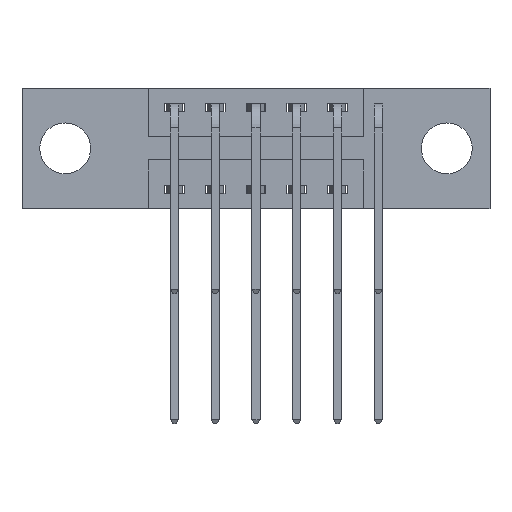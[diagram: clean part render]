
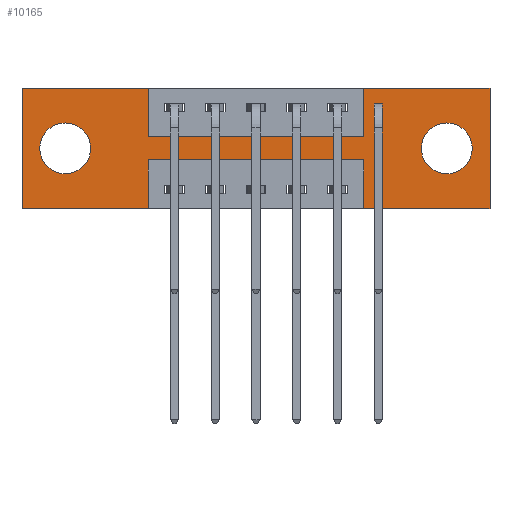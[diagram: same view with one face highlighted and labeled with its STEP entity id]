
A CAD part, front view. The second image highlights one B-rep face of the part: STEP entity #10165.
In plain terms, the highlighted planar face has unit normal (0, -1, 0).
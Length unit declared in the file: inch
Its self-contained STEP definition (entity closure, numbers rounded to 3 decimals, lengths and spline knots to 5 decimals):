
#234 = CARTESIAN_POINT ( 'NONE',  ( 0., 0., 0. ) ) ;
#360 = ORIENTED_EDGE ( 'NONE', *, *, #2505, .F. ) ;
#414 = DIRECTION ( 'NONE',  ( 0., 1., 0. ) ) ;
#424 = VECTOR ( 'NONE', #8199, 39.37008 ) ;
#481 = AXIS2_PLACEMENT_3D ( 'NONE', #708, #5631, #4730 ) ;
#499 = CIRCLE ( 'NONE', #2351, 0.078 ) ;
#577 = ORIENTED_EDGE ( 'NONE', *, *, #3240, .F. ) ;
#701 = ORIENTED_EDGE ( 'NONE', *, *, #3460, .T. ) ;
#708 = CARTESIAN_POINT ( 'NONE',  ( 0.1325, 0., -0.185 ) ) ;
#814 = EDGE_CURVE ( 'NONE', #5803, #1529, #7982, .T. ) ;
#855 = CARTESIAN_POINT ( 'NONE',  ( 0.3875, 0., 0. ) ) ;
#901 = ORIENTED_EDGE ( 'NONE', *, *, #8834, .F. ) ;
#1125 = EDGE_CURVE ( 'NONE', #2244, #5803, #10156, .T. ) ;
#1175 = DIRECTION ( 'NONE',  ( 0., 0., 1. ) ) ;
#1184 = DIRECTION ( 'NONE',  ( 1., 0., 0. ) ) ;
#1345 = DIRECTION ( 'NONE',  ( 0., 0., -1. ) ) ;
#1442 = CARTESIAN_POINT ( 'NONE',  ( 0.3875, 0., -0.37 ) ) ;
#1457 = CARTESIAN_POINT ( 'NONE',  ( 0.3875, 0., -0.15 ) ) ;
#1469 = CARTESIAN_POINT ( 'NONE',  ( 0., 0., 0. ) ) ;
#1529 = VERTEX_POINT ( 'NONE', #6823 ) ;
#1663 = CARTESIAN_POINT ( 'NONE',  ( 0., 0., -0.37 ) ) ;
#1689 = EDGE_LOOP ( 'NONE', ( #5128, #8986, #4815, #3028, #5295, #10006, #360, #7172, #8598, #577, #7775, #901 ) ) ;
#1960 = DIRECTION ( 'NONE',  ( 0., 1., 0. ) ) ;
#1968 = EDGE_CURVE ( 'NONE', #5763, #8391, #9096, .T. ) ;
#2097 = EDGE_CURVE ( 'NONE', #4335, #2244, #2822, .T. ) ;
#2244 = VERTEX_POINT ( 'NONE', #7338 ) ;
#2286 = EDGE_CURVE ( 'NONE', #3604, #5763, #9835, .T. ) ;
#2351 = AXIS2_PLACEMENT_3D ( 'NONE', #7688, #414, #3644 ) ;
#2410 = EDGE_LOOP ( 'NONE', ( #7696, #3784 ) ) ;
#2499 = VECTOR ( 'NONE', #6369, 39.37008 ) ;
#2505 = EDGE_CURVE ( 'NONE', #8391, #4384, #7104, .T. ) ;
#2518 = VECTOR ( 'NONE', #7050, 39.37008 ) ;
#2637 = VERTEX_POINT ( 'NONE', #1663 ) ;
#2639 = CARTESIAN_POINT ( 'NONE',  ( 0., 0., -0.37 ) ) ;
#2676 = VECTOR ( 'NONE', #4976, 39.37008 ) ;
#2822 = LINE ( 'NONE', #3824, #2499 ) ;
#2904 = VECTOR ( 'NONE', #5987, 39.37008 ) ;
#2987 = LINE ( 'NONE', #1442, #7530 ) ;
#3028 = ORIENTED_EDGE ( 'NONE', *, *, #1125, .F. ) ;
#3036 = CARTESIAN_POINT ( 'NONE',  ( 0.3875, 0., -0.22 ) ) ;
#3152 = CARTESIAN_POINT ( 'NONE',  ( 0., 0., -0.37 ) ) ;
#3240 = EDGE_CURVE ( 'NONE', #6927, #3604, #7519, .T. ) ;
#3460 = EDGE_CURVE ( 'NONE', #4185, #4206, #8150, .T. ) ;
#3530 = CARTESIAN_POINT ( 'NONE',  ( 1.3025, 0., -0.263 ) ) ;
#3537 = DIRECTION ( 'NONE',  ( -1., 0., 0. ) ) ;
#3566 = VECTOR ( 'NONE', #1184, 39.37008 ) ;
#3604 = VERTEX_POINT ( 'NONE', #5953 ) ;
#3644 = DIRECTION ( 'NONE',  ( 0., 0., -1. ) ) ;
#3784 = ORIENTED_EDGE ( 'NONE', *, *, #6646, .T. ) ;
#3816 = LINE ( 'NONE', #1469, #2518 ) ;
#3823 = CARTESIAN_POINT ( 'NONE',  ( 1.0475, 0., -0.37 ) ) ;
#3824 = CARTESIAN_POINT ( 'NONE',  ( 1.435, 0., 0. ) ) ;
#3940 = EDGE_LOOP ( 'NONE', ( #8589, #701 ) ) ;
#3952 = LINE ( 'NONE', #3152, #424 ) ;
#4122 = CARTESIAN_POINT ( 'NONE',  ( 0., 0., 0. ) ) ;
#4185 = VERTEX_POINT ( 'NONE', #3530 ) ;
#4206 = VERTEX_POINT ( 'NONE', #6722 ) ;
#4335 = VERTEX_POINT ( 'NONE', #9390 ) ;
#4384 = VERTEX_POINT ( 'NONE', #6299 ) ;
#4392 = LINE ( 'NONE', #10049, #2904 ) ;
#4565 = VECTOR ( 'NONE', #9618, 39.37008 ) ;
#4673 = AXIS2_PLACEMENT_3D ( 'NONE', #9257, #1960, #1175 ) ;
#4730 = DIRECTION ( 'NONE',  ( 0., 0., 1. ) ) ;
#4815 = ORIENTED_EDGE ( 'NONE', *, *, #814, .F. ) ;
#4856 = VECTOR ( 'NONE', #10333, 39.37008 ) ;
#4886 = DIRECTION ( 'NONE',  ( 0., 0., -1. ) ) ;
#4976 = DIRECTION ( 'NONE',  ( 0., 0., -1. ) ) ;
#5051 = CIRCLE ( 'NONE', #481, 0.078 ) ;
#5128 = ORIENTED_EDGE ( 'NONE', *, *, #7564, .F. ) ;
#5209 = VECTOR ( 'NONE', #3537, 39.37008 ) ;
#5295 = ORIENTED_EDGE ( 'NONE', *, *, #2097, .F. ) ;
#5406 = FACE_OUTER_BOUND ( 'NONE', #1689, .T. ) ;
#5475 = AXIS2_PLACEMENT_3D ( 'NONE', #7860, #8645, #10265 ) ;
#5510 = FACE_BOUND ( 'NONE', #2410, .T. ) ;
#5631 = DIRECTION ( 'NONE',  ( 0., 1., 0. ) ) ;
#5763 = VERTEX_POINT ( 'NONE', #1457 ) ;
#5803 = VERTEX_POINT ( 'NONE', #8009 ) ;
#5953 = CARTESIAN_POINT ( 'NONE',  ( 0.3875, 0., 0. ) ) ;
#5987 = DIRECTION ( 'NONE',  ( -1., 0., 0. ) ) ;
#6076 = EDGE_CURVE ( 'NONE', #2637, #6927, #9760, .T. ) ;
#6196 = CIRCLE ( 'NONE', #4673, 0.078 ) ;
#6202 = VECTOR ( 'NONE', #9002, 39.37008 ) ;
#6299 = CARTESIAN_POINT ( 'NONE',  ( 1.0475, 0., 0. ) ) ;
#6369 = DIRECTION ( 'NONE',  ( 0., 0., -1. ) ) ;
#6541 = DIRECTION ( 'NONE',  ( 0., 1., 0. ) ) ;
#6641 = VERTEX_POINT ( 'NONE', #7672 ) ;
#6646 = EDGE_CURVE ( 'NONE', #6641, #9813, #6196, .T. ) ;
#6722 = CARTESIAN_POINT ( 'NONE',  ( 1.3025, 0., -0.107 ) ) ;
#6823 = CARTESIAN_POINT ( 'NONE',  ( 1.0475, 0., -0.22 ) ) ;
#6927 = VERTEX_POINT ( 'NONE', #7342 ) ;
#6934 = CARTESIAN_POINT ( 'NONE',  ( 0.1325, 0., -0.107 ) ) ;
#6960 = AXIS2_PLACEMENT_3D ( 'NONE', #7240, #6541, #4886 ) ;
#7050 = DIRECTION ( 'NONE',  ( 1., 0., 0. ) ) ;
#7104 = LINE ( 'NONE', #7212, #4565 ) ;
#7172 = ORIENTED_EDGE ( 'NONE', *, *, #1968, .F. ) ;
#7212 = CARTESIAN_POINT ( 'NONE',  ( 1.0475, 0., 0. ) ) ;
#7240 = CARTESIAN_POINT ( 'NONE',  ( 1.3025, 0., -0.185 ) ) ;
#7338 = CARTESIAN_POINT ( 'NONE',  ( 1.435, 0., -0.37 ) ) ;
#7342 = CARTESIAN_POINT ( 'NONE',  ( 0., 0., 0. ) ) ;
#7375 = CARTESIAN_POINT ( 'NONE',  ( 1.0475, 0., -0.15 ) ) ;
#7418 = CARTESIAN_POINT ( 'NONE',  ( 0.3875, 0., -0.15 ) ) ;
#7519 = LINE ( 'NONE', #234, #3566 ) ;
#7530 = VECTOR ( 'NONE', #1345, 39.37008 ) ;
#7564 = EDGE_CURVE ( 'NONE', #9030, #8965, #2987, .T. ) ;
#7672 = CARTESIAN_POINT ( 'NONE',  ( 0.1325, 0., -0.263 ) ) ;
#7688 = CARTESIAN_POINT ( 'NONE',  ( 1.3025, 0., -0.185 ) ) ;
#7696 = ORIENTED_EDGE ( 'NONE', *, *, #9245, .T. ) ;
#7775 = ORIENTED_EDGE ( 'NONE', *, *, #6076, .F. ) ;
#7860 = CARTESIAN_POINT ( 'NONE',  ( 0., 0., -0.37 ) ) ;
#7982 = LINE ( 'NONE', #3823, #4856 ) ;
#8009 = CARTESIAN_POINT ( 'NONE',  ( 1.0475, 0., -0.37 ) ) ;
#8150 = CIRCLE ( 'NONE', #6960, 0.078 ) ;
#8199 = DIRECTION ( 'NONE',  ( -1., 0., 0. ) ) ;
#8391 = VERTEX_POINT ( 'NONE', #7375 ) ;
#8589 = ORIENTED_EDGE ( 'NONE', *, *, #10518, .T. ) ;
#8598 = ORIENTED_EDGE ( 'NONE', *, *, #2286, .F. ) ;
#8645 = DIRECTION ( 'NONE',  ( 0., -1., 0. ) ) ;
#8754 = PLANE ( 'NONE',  #5475 ) ;
#8834 = EDGE_CURVE ( 'NONE', #8965, #2637, #3952, .T. ) ;
#8965 = VERTEX_POINT ( 'NONE', #9265 ) ;
#8986 = ORIENTED_EDGE ( 'NONE', *, *, #9998, .F. ) ;
#9002 = DIRECTION ( 'NONE',  ( 0., 0., 1. ) ) ;
#9030 = VERTEX_POINT ( 'NONE', #3036 ) ;
#9096 = LINE ( 'NONE', #7418, #10170 ) ;
#9245 = EDGE_CURVE ( 'NONE', #9813, #6641, #5051, .T. ) ;
#9257 = CARTESIAN_POINT ( 'NONE',  ( 0.1325, 0., -0.185 ) ) ;
#9265 = CARTESIAN_POINT ( 'NONE',  ( 0.3875, 0., -0.37 ) ) ;
#9390 = CARTESIAN_POINT ( 'NONE',  ( 1.435, 0., 0. ) ) ;
#9452 = FACE_BOUND ( 'NONE', #3940, .T. ) ;
#9496 = EDGE_CURVE ( 'NONE', #4384, #4335, #3816, .T. ) ;
#9618 = DIRECTION ( 'NONE',  ( 0., 0., 1. ) ) ;
#9760 = LINE ( 'NONE', #4122, #6202 ) ;
#9813 = VERTEX_POINT ( 'NONE', #6934 ) ;
#9835 = LINE ( 'NONE', #855, #2676 ) ;
#9857 = DIRECTION ( 'NONE',  ( 1., 0., 0. ) ) ;
#9998 = EDGE_CURVE ( 'NONE', #1529, #9030, #4392, .T. ) ;
#10006 = ORIENTED_EDGE ( 'NONE', *, *, #9496, .F. ) ;
#10049 = CARTESIAN_POINT ( 'NONE',  ( 0.3875, 0., -0.22 ) ) ;
#10156 = LINE ( 'NONE', #2639, #5209 ) ;
#10165 = ADVANCED_FACE ( 'NONE', ( #9452, #5510, #5406 ), #8754, .T. ) ;
#10170 = VECTOR ( 'NONE', #9857, 39.37008 ) ;
#10265 = DIRECTION ( 'NONE',  ( 0., 0., -1. ) ) ;
#10333 = DIRECTION ( 'NONE',  ( 0., 0., 1. ) ) ;
#10518 = EDGE_CURVE ( 'NONE', #4206, #4185, #499, .T. ) ;
